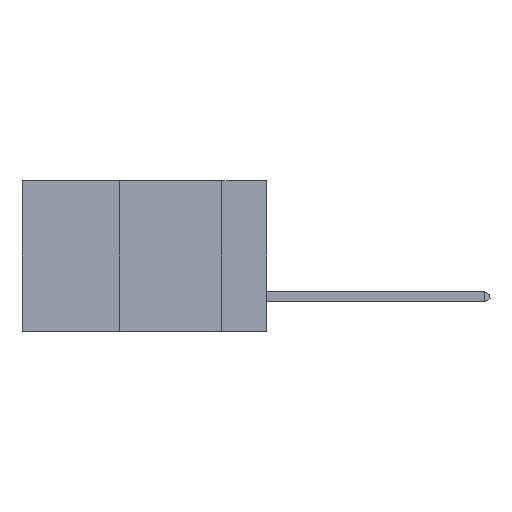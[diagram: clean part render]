
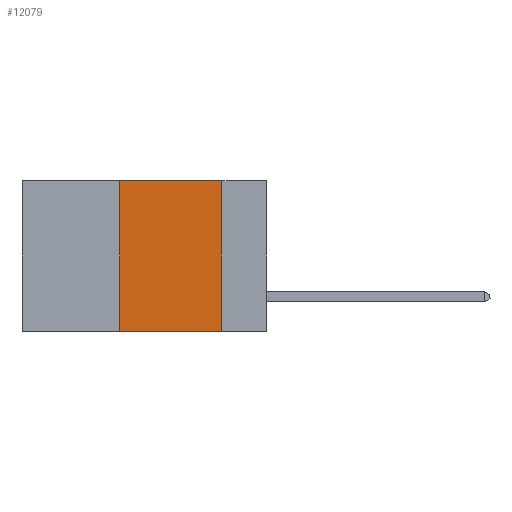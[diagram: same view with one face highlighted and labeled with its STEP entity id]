
A CAD part, left-side view. The second image highlights one B-rep face of the part: STEP entity #12079.
In plain terms, the highlighted planar face has unit normal (-1, 0, 0).
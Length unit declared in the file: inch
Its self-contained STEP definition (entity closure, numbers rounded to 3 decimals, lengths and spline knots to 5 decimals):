
#19 = DIRECTION ( 'NONE',  ( 0., 0., -1. ) ) ;
#793 = CARTESIAN_POINT ( 'NONE',  ( 0., 0.6, -0.37 ) ) ;
#1461 = DIRECTION ( 'NONE',  ( 0., 0., 1. ) ) ;
#2041 = ORIENTED_EDGE ( 'NONE', *, *, #2498, .F. ) ;
#2093 = ORIENTED_EDGE ( 'NONE', *, *, #8693, .F. ) ;
#2258 = CARTESIAN_POINT ( 'NONE',  ( 0., 0.11, 0. ) ) ;
#2498 = EDGE_CURVE ( 'NONE', #6081, #9136, #5040, .T. ) ;
#2548 = ORIENTED_EDGE ( 'NONE', *, *, #7453, .T. ) ;
#3114 = VECTOR ( 'NONE', #1461, 39.37008 ) ;
#3474 = ORIENTED_EDGE ( 'NONE', *, *, #7920, .F. ) ;
#4229 = CARTESIAN_POINT ( 'NONE',  ( 0., 0.36, -0.37 ) ) ;
#5040 = LINE ( 'NONE', #8100, #7576 ) ;
#5152 = PLANE ( 'NONE',  #9900 ) ;
#5463 = CARTESIAN_POINT ( 'NONE',  ( 0., 0.11, -0.37 ) ) ;
#5514 = VERTEX_POINT ( 'NONE', #5463 ) ;
#6081 = VERTEX_POINT ( 'NONE', #11666 ) ;
#6164 = DIRECTION ( 'NONE',  ( 1., 0., 0. ) ) ;
#6529 = CARTESIAN_POINT ( 'NONE',  ( 0., 0.36, 0. ) ) ;
#7101 = EDGE_LOOP ( 'NONE', ( #2093, #2041, #3474, #2548 ) ) ;
#7396 = CARTESIAN_POINT ( 'NONE',  ( 0., 0.11, 0. ) ) ;
#7453 = EDGE_CURVE ( 'NONE', #10545, #5514, #10339, .T. ) ;
#7553 = VECTOR ( 'NONE', #8274, 39.37008 ) ;
#7576 = VECTOR ( 'NONE', #9467, 39.37008 ) ;
#7920 = EDGE_CURVE ( 'NONE', #10545, #6081, #8553, .T. ) ;
#8100 = CARTESIAN_POINT ( 'NONE',  ( 0., 0.6, 0. ) ) ;
#8274 = DIRECTION ( 'NONE',  ( 0., 0., -1. ) ) ;
#8533 = VECTOR ( 'NONE', #10384, 39.37008 ) ;
#8553 = LINE ( 'NONE', #6529, #3114 ) ;
#8693 = EDGE_CURVE ( 'NONE', #9136, #5514, #10165, .T. ) ;
#8699 = FACE_OUTER_BOUND ( 'NONE', #7101, .T. ) ;
#9136 = VERTEX_POINT ( 'NONE', #2258 ) ;
#9467 = DIRECTION ( 'NONE',  ( 0., -1., 0. ) ) ;
#9900 = AXIS2_PLACEMENT_3D ( 'NONE', #11531, #6164, #19 ) ;
#10165 = LINE ( 'NONE', #7396, #7553 ) ;
#10339 = LINE ( 'NONE', #793, #8533 ) ;
#10384 = DIRECTION ( 'NONE',  ( 0., -1., 0. ) ) ;
#10545 = VERTEX_POINT ( 'NONE', #4229 ) ;
#11531 = CARTESIAN_POINT ( 'NONE',  ( 0., 0.6, 0. ) ) ;
#11666 = CARTESIAN_POINT ( 'NONE',  ( 0., 0.36, 0. ) ) ;
#12079 = ADVANCED_FACE ( 'NONE', ( #8699 ), #5152, .F. ) ;
